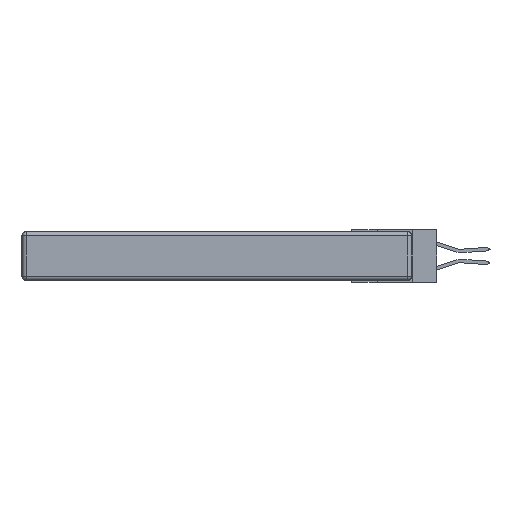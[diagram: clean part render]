
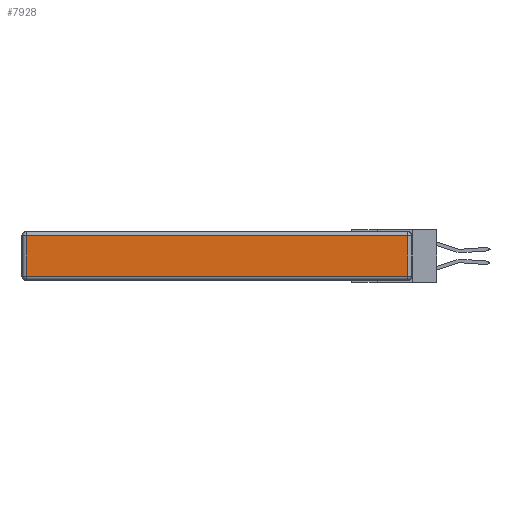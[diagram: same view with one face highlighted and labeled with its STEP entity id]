
A CAD part, left-side view. The second image highlights one B-rep face of the part: STEP entity #7928.
In plain terms, the highlighted planar face has unit normal (-1, 0, 0).
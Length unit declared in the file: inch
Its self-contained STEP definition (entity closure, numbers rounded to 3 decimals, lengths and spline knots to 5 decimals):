
#36 = CARTESIAN_POINT ( 'NONE',  ( 0., 0., -0.313 ) ) ;
#741 = CARTESIAN_POINT ( 'NONE',  ( 0., 2.72, -0.03 ) ) ;
#1607 = VECTOR ( 'NONE', #33705, 39.37008 ) ;
#1693 = CARTESIAN_POINT ( 'NONE',  ( 0., 0.03, -0.343 ) ) ;
#2025 = CARTESIAN_POINT ( 'NONE',  ( 0., 2.75, -0.03 ) ) ;
#2685 = VERTEX_POINT ( 'NONE', #4667 ) ;
#3946 = AXIS2_PLACEMENT_3D ( 'NONE', #25587, #9615, #22704 ) ;
#4667 = CARTESIAN_POINT ( 'NONE',  ( 0., 0.03, -0.313 ) ) ;
#5435 = ORIENTED_EDGE ( 'NONE', *, *, #23591, .T. ) ;
#5766 = LINE ( 'NONE', #1693, #13604 ) ;
#6578 = CARTESIAN_POINT ( 'NONE',  ( 0., 2.72, -0.343 ) ) ;
#7073 = LINE ( 'NONE', #6578, #31115 ) ;
#7928 = ADVANCED_FACE ( 'NONE', ( #27592 ), #12019, .T. ) ;
#9615 = DIRECTION ( 'NONE',  ( -1., 0., 0. ) ) ;
#12019 = PLANE ( 'NONE',  #3946 ) ;
#13604 = VECTOR ( 'NONE', #22505, 39.37008 ) ;
#15123 = LINE ( 'NONE', #36, #21321 ) ;
#15930 = ORIENTED_EDGE ( 'NONE', *, *, #28269, .T. ) ;
#17737 = LINE ( 'NONE', #2025, #1607 ) ;
#18888 = VERTEX_POINT ( 'NONE', #24297 ) ;
#19803 = EDGE_LOOP ( 'NONE', ( #28840, #23299, #5435, #15930 ) ) ;
#21321 = VECTOR ( 'NONE', #31758, 39.37008 ) ;
#22505 = DIRECTION ( 'NONE',  ( 0., 0., 1. ) ) ;
#22704 = DIRECTION ( 'NONE',  ( 0., 0., 1. ) ) ;
#23299 = ORIENTED_EDGE ( 'NONE', *, *, #30981, .T. ) ;
#23464 = CARTESIAN_POINT ( 'NONE',  ( 0., 0.03, -0.03 ) ) ;
#23591 = EDGE_CURVE ( 'NONE', #30646, #31653, #17737, .T. ) ;
#24297 = CARTESIAN_POINT ( 'NONE',  ( 0., 2.72, -0.313 ) ) ;
#25587 = CARTESIAN_POINT ( 'NONE',  ( 0., 0., -0.343 ) ) ;
#25770 = EDGE_CURVE ( 'NONE', #18888, #2685, #15123, .T. ) ;
#27592 = FACE_OUTER_BOUND ( 'NONE', #19803, .T. ) ;
#28269 = EDGE_CURVE ( 'NONE', #31653, #18888, #7073, .T. ) ;
#28840 = ORIENTED_EDGE ( 'NONE', *, *, #25770, .T. ) ;
#30441 = DIRECTION ( 'NONE',  ( 0., 0., -1. ) ) ;
#30646 = VERTEX_POINT ( 'NONE', #23464 ) ;
#30981 = EDGE_CURVE ( 'NONE', #2685, #30646, #5766, .T. ) ;
#31115 = VECTOR ( 'NONE', #30441, 39.37008 ) ;
#31653 = VERTEX_POINT ( 'NONE', #741 ) ;
#31758 = DIRECTION ( 'NONE',  ( 0., -1., 0. ) ) ;
#33705 = DIRECTION ( 'NONE',  ( 0., 1., 0. ) ) ;
